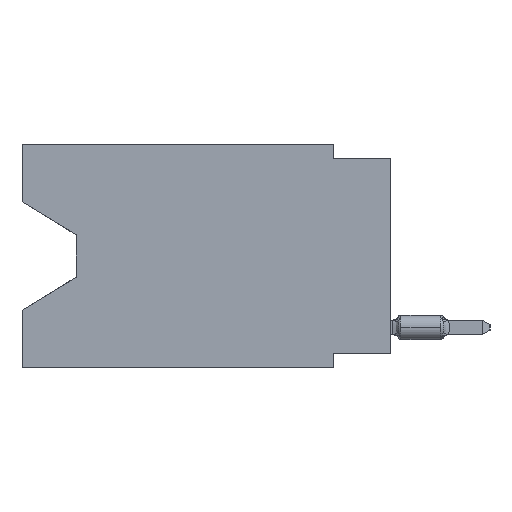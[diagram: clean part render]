
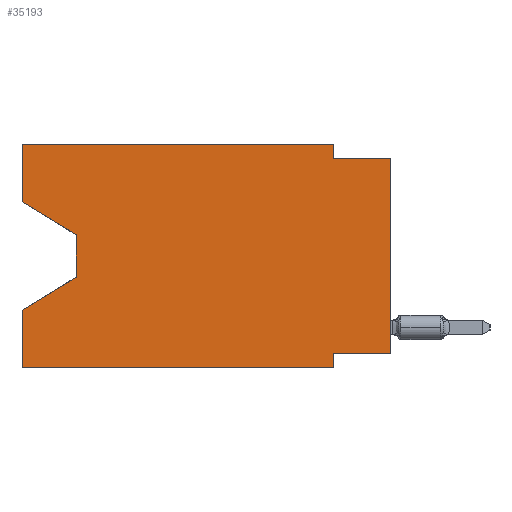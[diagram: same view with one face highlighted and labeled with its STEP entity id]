
A CAD part, left-side view. The second image highlights one B-rep face of the part: STEP entity #35193.
In plain terms, the highlighted planar face has unit normal (-1, 0, 0).
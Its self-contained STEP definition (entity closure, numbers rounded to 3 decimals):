
#680 = AXIS2_PLACEMENT_3D ( 'NONE', #3303, #76462, #52587 ) ;
#1392 = LINE ( 'NONE', #14323, #74018 ) ;
#2543 = EDGE_CURVE ( 'NONE', #62002, #47695, #11874, .T. ) ;
#2603 = VERTEX_POINT ( 'NONE', #55106 ) ;
#3303 = CARTESIAN_POINT ( 'NONE',  ( 0., 16.383, 0. ) ) ;
#5056 = CARTESIAN_POINT ( 'NONE',  ( 0., 16.383, -2.546 ) ) ;
#7007 = VERTEX_POINT ( 'NONE', #8228 ) ;
#7387 = VERTEX_POINT ( 'NONE', #14195 ) ;
#8228 = CARTESIAN_POINT ( 'NONE',  ( 0., 16.383, -9.906 ) ) ;
#8456 = CARTESIAN_POINT ( 'NONE',  ( 0., 16.383, -9.906 ) ) ;
#8588 = LINE ( 'NONE', #46933, #52044 ) ;
#9265 = VECTOR ( 'NONE', #68979, 1000. ) ;
#10377 = EDGE_LOOP ( 'NONE', ( #54162, #76735, #17993, #43545, #70323, #74967, #34586, #50570, #48913, #33097, #74416, #17638 ) ) ;
#10737 = CARTESIAN_POINT ( 'NONE',  ( 0., 0., 0. ) ) ;
#11874 = LINE ( 'NONE', #67621, #62265 ) ;
#12040 = CARTESIAN_POINT ( 'NONE',  ( 0., 16.383, 0. ) ) ;
#12357 = VERTEX_POINT ( 'NONE', #36940 ) ;
#13370 = LINE ( 'NONE', #56593, #38474 ) ;
#13643 = VECTOR ( 'NONE', #54870, 1000. ) ;
#13729 = LINE ( 'NONE', #8456, #22608 ) ;
#14195 = CARTESIAN_POINT ( 'NONE',  ( 0., 16.383, -2.546 ) ) ;
#14323 = CARTESIAN_POINT ( 'NONE',  ( 0., 16.383, 0. ) ) ;
#14745 = CARTESIAN_POINT ( 'NONE',  ( 0., 2.54, -9.906 ) ) ;
#15105 = DIRECTION ( 'NONE',  ( 0., 0., -1. ) ) ;
#16629 = FACE_OUTER_BOUND ( 'NONE', #10377, .T. ) ;
#17638 = ORIENTED_EDGE ( 'NONE', *, *, #44322, .F. ) ;
#17736 = VERTEX_POINT ( 'NONE', #22134 ) ;
#17856 = DIRECTION ( 'NONE',  ( 0., 0., -1. ) ) ;
#17993 = ORIENTED_EDGE ( 'NONE', *, *, #25752, .T. ) ;
#19699 = CARTESIAN_POINT ( 'NONE',  ( 0., 2.54, -9.906 ) ) ;
#19985 = DIRECTION ( 'NONE',  ( 0., 0., 1. ) ) ;
#20577 = DIRECTION ( 'NONE',  ( 0., -1., 0. ) ) ;
#21886 = DIRECTION ( 'NONE',  ( 0., 0., 1. ) ) ;
#21968 = CARTESIAN_POINT ( 'NONE',  ( 0., 2.54, 0. ) ) ;
#22134 = CARTESIAN_POINT ( 'NONE',  ( 0., 13.97, -5.893 ) ) ;
#22496 = DIRECTION ( 'NONE',  ( 0., -1., 0. ) ) ;
#22608 = VECTOR ( 'NONE', #20577, 1000. ) ;
#23596 = EDGE_CURVE ( 'NONE', #2603, #17736, #70439, .T. ) ;
#24557 = EDGE_CURVE ( 'NONE', #62002, #12357, #65674, .T. ) ;
#25752 = EDGE_CURVE ( 'NONE', #17736, #26654, #61275, .T. ) ;
#26654 = VERTEX_POINT ( 'NONE', #31528 ) ;
#26746 = CARTESIAN_POINT ( 'NONE',  ( 0., 16.383, 0. ) ) ;
#26868 = CARTESIAN_POINT ( 'NONE',  ( 0., 2.54, -0.635 ) ) ;
#28559 = VECTOR ( 'NONE', #15105, 1000. ) ;
#28579 = CARTESIAN_POINT ( 'NONE',  ( 0., 0., -9.271 ) ) ;
#29017 = EDGE_CURVE ( 'NONE', #7387, #2603, #78602, .T. ) ;
#29868 = VECTOR ( 'NONE', #41815, 1000. ) ;
#30542 = CARTESIAN_POINT ( 'NONE',  ( 0., 13.97, -5.893 ) ) ;
#31528 = CARTESIAN_POINT ( 'NONE',  ( 0., 16.383, -7.36 ) ) ;
#32688 = VECTOR ( 'NONE', #22496, 1000. ) ;
#33097 = ORIENTED_EDGE ( 'NONE', *, *, #73658, .F. ) ;
#33320 = EDGE_CURVE ( 'NONE', #38239, #12357, #79078, .T. ) ;
#33526 = VERTEX_POINT ( 'NONE', #14745 ) ;
#33647 = VERTEX_POINT ( 'NONE', #21968 ) ;
#34586 = ORIENTED_EDGE ( 'NONE', *, *, #2543, .F. ) ;
#35193 = ADVANCED_FACE ( 'NONE', ( #16629 ), #46932, .F. ) ;
#35364 = DIRECTION ( 'NONE',  ( 0., 0., 1. ) ) ;
#35677 = VECTOR ( 'NONE', #35364, 1000. ) ;
#36940 = CARTESIAN_POINT ( 'NONE',  ( 0., 0., -0.635 ) ) ;
#37807 = DIRECTION ( 'NONE',  ( 0., 0.855, -0.519 ) ) ;
#38239 = VERTEX_POINT ( 'NONE', #26868 ) ;
#38474 = VECTOR ( 'NONE', #17856, 1000. ) ;
#41815 = DIRECTION ( 'NONE',  ( 0., -0.855, -0.519 ) ) ;
#42211 = EDGE_CURVE ( 'NONE', #47695, #33526, #76256, .T. ) ;
#43545 = ORIENTED_EDGE ( 'NONE', *, *, #69518, .F. ) ;
#44322 = EDGE_CURVE ( 'NONE', #7387, #65795, #8588, .T. ) ;
#46932 = PLANE ( 'NONE',  #680 ) ;
#46933 = CARTESIAN_POINT ( 'NONE',  ( 0., 16.383, 0. ) ) ;
#47695 = VERTEX_POINT ( 'NONE', #57864 ) ;
#48913 = ORIENTED_EDGE ( 'NONE', *, *, #33320, .F. ) ;
#50570 = ORIENTED_EDGE ( 'NONE', *, *, #24557, .T. ) ;
#52044 = VECTOR ( 'NONE', #21886, 1000. ) ;
#52587 = DIRECTION ( 'NONE',  ( 0., 0., -1. ) ) ;
#53612 = CARTESIAN_POINT ( 'NONE',  ( 0., 0., -0.635 ) ) ;
#53919 = EDGE_CURVE ( 'NONE', #7007, #33526, #13729, .T. ) ;
#54162 = ORIENTED_EDGE ( 'NONE', *, *, #29017, .T. ) ;
#54180 = EDGE_CURVE ( 'NONE', #65795, #33647, #67774, .T. ) ;
#54870 = DIRECTION ( 'NONE',  ( 0., -1., 0. ) ) ;
#55106 = CARTESIAN_POINT ( 'NONE',  ( 0., 13.97, -4.013 ) ) ;
#56593 = CARTESIAN_POINT ( 'NONE',  ( 0., 2.54, 0. ) ) ;
#57530 = CARTESIAN_POINT ( 'NONE',  ( 0., 13.97, -4.013 ) ) ;
#57864 = CARTESIAN_POINT ( 'NONE',  ( 0., 2.54, -9.271 ) ) ;
#61275 = LINE ( 'NONE', #30542, #71897 ) ;
#62002 = VERTEX_POINT ( 'NONE', #28579 ) ;
#62265 = VECTOR ( 'NONE', #79757, 1000. ) ;
#65674 = LINE ( 'NONE', #10737, #35677 ) ;
#65795 = VERTEX_POINT ( 'NONE', #26746 ) ;
#67621 = CARTESIAN_POINT ( 'NONE',  ( 0., 0., -9.271 ) ) ;
#67774 = LINE ( 'NONE', #12040, #13643 ) ;
#68979 = DIRECTION ( 'NONE',  ( 0., 0., -1. ) ) ;
#69518 = EDGE_CURVE ( 'NONE', #7007, #26654, #1392, .T. ) ;
#70323 = ORIENTED_EDGE ( 'NONE', *, *, #53919, .T. ) ;
#70439 = LINE ( 'NONE', #57530, #28559 ) ;
#71897 = VECTOR ( 'NONE', #37807, 1000. ) ;
#73658 = EDGE_CURVE ( 'NONE', #33647, #38239, #13370, .T. ) ;
#74018 = VECTOR ( 'NONE', #19985, 1000. ) ;
#74416 = ORIENTED_EDGE ( 'NONE', *, *, #54180, .F. ) ;
#74967 = ORIENTED_EDGE ( 'NONE', *, *, #42211, .F. ) ;
#76256 = LINE ( 'NONE', #19699, #9265 ) ;
#76462 = DIRECTION ( 'NONE',  ( 1., 0., 0. ) ) ;
#76735 = ORIENTED_EDGE ( 'NONE', *, *, #23596, .T. ) ;
#78602 = LINE ( 'NONE', #5056, #29868 ) ;
#79078 = LINE ( 'NONE', #53612, #32688 ) ;
#79757 = DIRECTION ( 'NONE',  ( 0., 1., 0. ) ) ;
